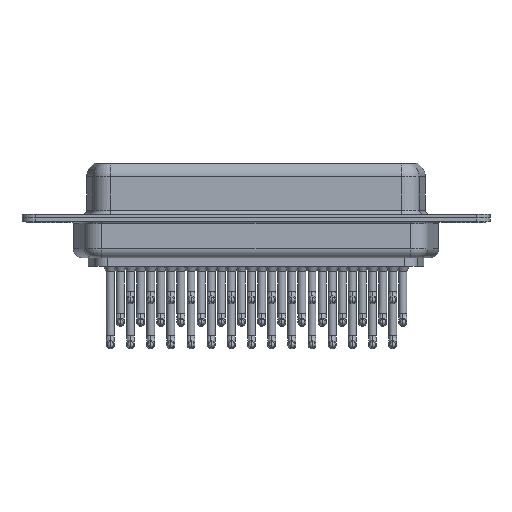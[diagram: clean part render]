
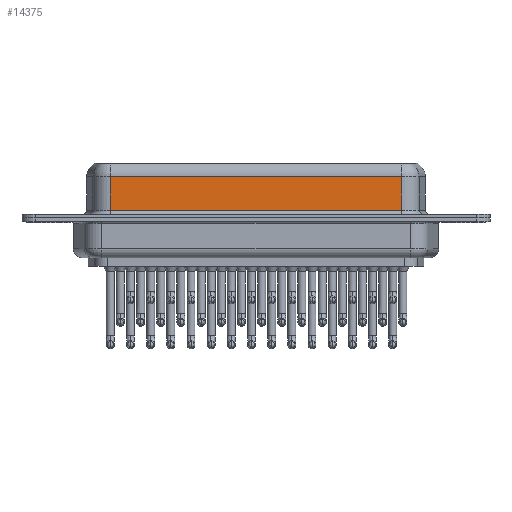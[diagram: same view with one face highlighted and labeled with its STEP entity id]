
A CAD part, front view. The second image highlights one B-rep face of the part: STEP entity #14375.
In plain terms, the highlighted planar face has unit normal (0, -1, 0).
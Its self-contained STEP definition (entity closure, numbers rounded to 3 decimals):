
#505 = ORIENTED_EDGE ( 'NONE', *, *, #2652, .T. ) ;
#523 = CARTESIAN_POINT ( 'NONE',  ( 7.013, -3.95, 6.4 ) ) ;
#2652 = EDGE_CURVE ( 'NONE', #9230, #7548, #6433, .T. ) ;
#2654 = DIRECTION ( 'NONE',  ( 0., 0., -1. ) ) ;
#4284 = LINE ( 'NONE', #24769, #27497 ) ;
#4798 = ORIENTED_EDGE ( 'NONE', *, *, #15088, .T. ) ;
#5405 = FACE_OUTER_BOUND ( 'NONE', #23805, .T. ) ;
#5544 = LINE ( 'NONE', #17549, #10728 ) ;
#5793 = DIRECTION ( 'NONE',  ( -1., 0., 0. ) ) ;
#6433 = LINE ( 'NONE', #523, #7121 ) ;
#6567 = CARTESIAN_POINT ( 'NONE',  ( 40.037, -3.95, 0.9 ) ) ;
#6614 = CARTESIAN_POINT ( 'NONE',  ( 7.013, -3.95, 0.9 ) ) ;
#7121 = VECTOR ( 'NONE', #2654, 1000. ) ;
#7269 = ORIENTED_EDGE ( 'NONE', *, *, #7474, .T. ) ;
#7368 = CARTESIAN_POINT ( 'NONE',  ( 7.013, -3.95, 4.65 ) ) ;
#7474 = EDGE_CURVE ( 'NONE', #7548, #16487, #5544, .T. ) ;
#7548 = VERTEX_POINT ( 'NONE', #6614 ) ;
#8144 = VECTOR ( 'NONE', #5793, 1000. ) ;
#9230 = VERTEX_POINT ( 'NONE', #7368 ) ;
#9571 = CARTESIAN_POINT ( 'NONE',  ( 40.037, -3.95, 6.4 ) ) ;
#10728 = VECTOR ( 'NONE', #26604, 1000. ) ;
#11207 = DIRECTION ( 'NONE',  ( 0., 0., -1. ) ) ;
#11822 = DIRECTION ( 'NONE',  ( 0., 0., 1. ) ) ;
#12979 = CARTESIAN_POINT ( 'NONE',  ( 40.037, -3.95, 4.65 ) ) ;
#13463 = ORIENTED_EDGE ( 'NONE', *, *, #16566, .F. ) ;
#14375 = ADVANCED_FACE ( 'NONE', ( #5405 ), #25288, .F. ) ;
#15088 = EDGE_CURVE ( 'NONE', #21142, #9230, #20103, .T. ) ;
#16487 = VERTEX_POINT ( 'NONE', #6567 ) ;
#16566 = EDGE_CURVE ( 'NONE', #21142, #16487, #4284, .T. ) ;
#17549 = CARTESIAN_POINT ( 'NONE',  ( 40.037, -3.95, 0.9 ) ) ;
#18499 = AXIS2_PLACEMENT_3D ( 'NONE', #9571, #25382, #11822 ) ;
#19183 = CARTESIAN_POINT ( 'NONE',  ( 40.037, -3.95, 4.65 ) ) ;
#20103 = LINE ( 'NONE', #19183, #8144 ) ;
#21142 = VERTEX_POINT ( 'NONE', #12979 ) ;
#23805 = EDGE_LOOP ( 'NONE', ( #13463, #4798, #505, #7269 ) ) ;
#24769 = CARTESIAN_POINT ( 'NONE',  ( 40.037, -3.95, 6.4 ) ) ;
#25288 = PLANE ( 'NONE',  #18499 ) ;
#25382 = DIRECTION ( 'NONE',  ( 0., 1., 0. ) ) ;
#26604 = DIRECTION ( 'NONE',  ( 1., 0., 0. ) ) ;
#27497 = VECTOR ( 'NONE', #11207, 1000. ) ;
